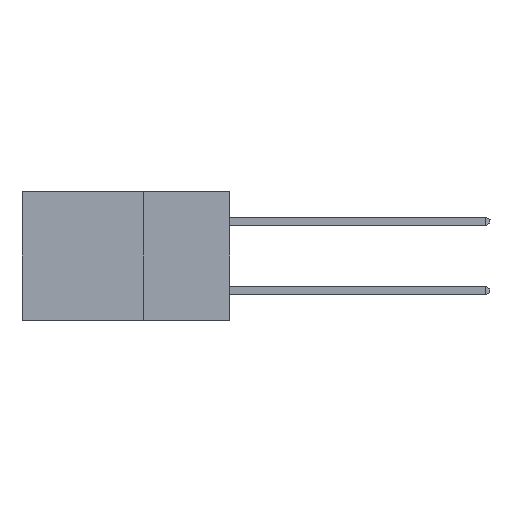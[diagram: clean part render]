
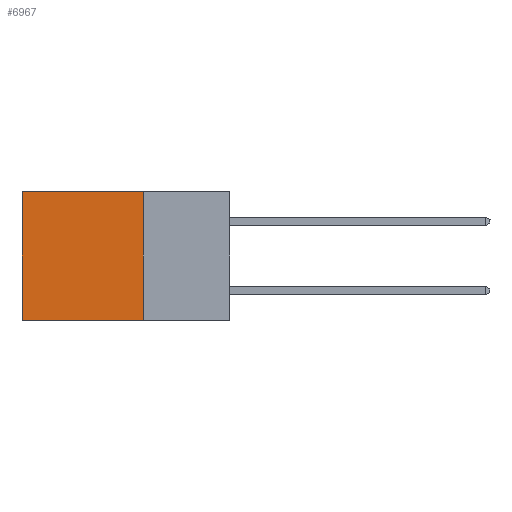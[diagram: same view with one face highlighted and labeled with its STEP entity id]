
A CAD part, left-side view. The second image highlights one B-rep face of the part: STEP entity #6967.
In plain terms, the highlighted planar face has unit normal (-1, 0, 0).
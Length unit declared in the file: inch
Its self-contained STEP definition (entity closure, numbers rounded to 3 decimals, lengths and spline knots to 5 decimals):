
#599 = CARTESIAN_POINT ( 'NONE',  ( 0.298, 0.6, 0. ) ) ;
#787 = EDGE_LOOP ( 'NONE', ( #7123, #9887, #7781, #9006 ) ) ;
#1396 = VERTEX_POINT ( 'NONE', #9984 ) ;
#1563 = VERTEX_POINT ( 'NONE', #9494 ) ;
#1959 = VECTOR ( 'NONE', #2328, 39.37008 ) ;
#2077 = PLANE ( 'NONE',  #6125 ) ;
#2114 = LINE ( 'NONE', #9002, #1959 ) ;
#2328 = DIRECTION ( 'NONE',  ( 0., 1., 0. ) ) ;
#2674 = DIRECTION ( 'NONE',  ( 0., 0., -1. ) ) ;
#3493 = EDGE_CURVE ( 'NONE', #11775, #12258, #10741, .T. ) ;
#5201 = CARTESIAN_POINT ( 'NONE',  ( 0.298, 0.25, -0.37 ) ) ;
#5205 = EDGE_CURVE ( 'NONE', #11775, #1563, #9625, .T. ) ;
#6048 = VECTOR ( 'NONE', #2674, 39.37008 ) ;
#6125 = AXIS2_PLACEMENT_3D ( 'NONE', #10046, #8138, #9104 ) ;
#6487 = VECTOR ( 'NONE', #11140, 39.37008 ) ;
#6967 = ADVANCED_FACE ( 'NONE', ( #8629 ), #2077, .F. ) ;
#6978 = LINE ( 'NONE', #599, #6048 ) ;
#7123 = ORIENTED_EDGE ( 'NONE', *, *, #12837, .T. ) ;
#7781 = ORIENTED_EDGE ( 'NONE', *, *, #3493, .F. ) ;
#8138 = DIRECTION ( 'NONE',  ( 1., 0., 0. ) ) ;
#8629 = FACE_OUTER_BOUND ( 'NONE', #787, .T. ) ;
#8923 = CARTESIAN_POINT ( 'NONE',  ( 0.298, 0.25, 0. ) ) ;
#9002 = CARTESIAN_POINT ( 'NONE',  ( 0.298, 0.25, -0.37 ) ) ;
#9006 = ORIENTED_EDGE ( 'NONE', *, *, #5205, .T. ) ;
#9104 = DIRECTION ( 'NONE',  ( 0., 0., -1. ) ) ;
#9494 = CARTESIAN_POINT ( 'NONE',  ( 0.298, 0.6, 0. ) ) ;
#9625 = LINE ( 'NONE', #10633, #11846 ) ;
#9887 = ORIENTED_EDGE ( 'NONE', *, *, #12562, .F. ) ;
#9984 = CARTESIAN_POINT ( 'NONE',  ( 0.298, 0.6, -0.37 ) ) ;
#10046 = CARTESIAN_POINT ( 'NONE',  ( 0.298, 0.25, 0. ) ) ;
#10121 = CARTESIAN_POINT ( 'NONE',  ( 0.298, 0.25, 0. ) ) ;
#10633 = CARTESIAN_POINT ( 'NONE',  ( 0.298, 0.25, 0. ) ) ;
#10741 = LINE ( 'NONE', #10121, #6487 ) ;
#11140 = DIRECTION ( 'NONE',  ( 0., 0., -1. ) ) ;
#11567 = DIRECTION ( 'NONE',  ( 0., 1., 0. ) ) ;
#11775 = VERTEX_POINT ( 'NONE', #8923 ) ;
#11846 = VECTOR ( 'NONE', #11567, 39.37008 ) ;
#12258 = VERTEX_POINT ( 'NONE', #5201 ) ;
#12562 = EDGE_CURVE ( 'NONE', #12258, #1396, #2114, .T. ) ;
#12837 = EDGE_CURVE ( 'NONE', #1563, #1396, #6978, .T. ) ;
